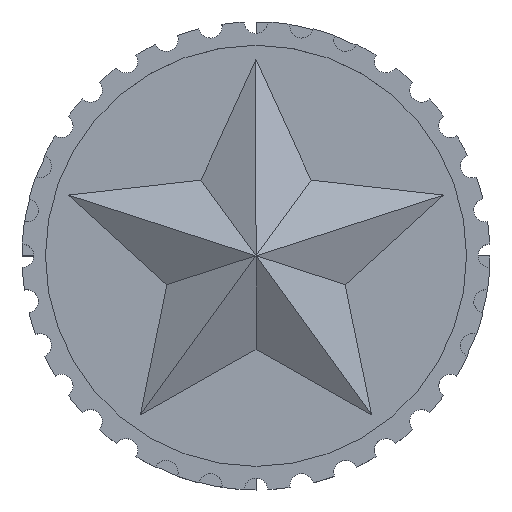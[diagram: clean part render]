
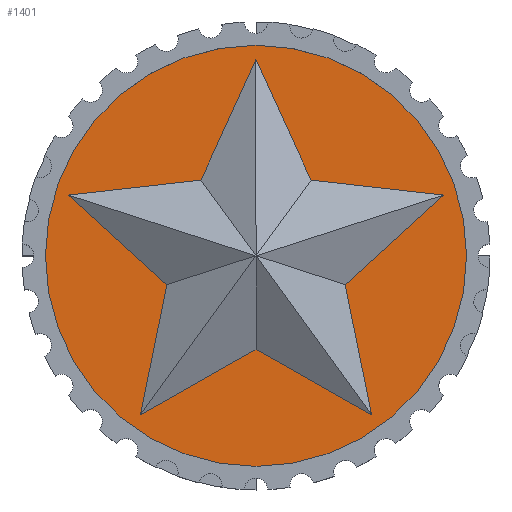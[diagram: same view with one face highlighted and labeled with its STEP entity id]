
A CAD part, top view. The second image highlights one B-rep face of the part: STEP entity #1401.
In plain terms, the highlighted planar face has unit normal (0, 0, 1).
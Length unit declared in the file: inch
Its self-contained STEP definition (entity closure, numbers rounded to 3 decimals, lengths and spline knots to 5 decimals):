
#27 = EDGE_CURVE ( 'NONE', #3067, #228, #1392, .T. ) ;
#35 = VERTEX_POINT ( 'NONE', #1314 ) ;
#119 = EDGE_CURVE ( 'NONE', #2326, #4335, #679, .T. ) ;
#147 = ORIENTED_EDGE ( 'NONE', *, *, #1856, .F. ) ;
#154 = EDGE_CURVE ( 'NONE', #560, #3881, #2661, .T. ) ;
#228 = VERTEX_POINT ( 'NONE', #1387 ) ;
#315 = LINE ( 'NONE', #2724, #3846 ) ;
#325 = CARTESIAN_POINT ( 'NONE',  ( 0., -0.25, 0.26063 ) ) ;
#347 = ORIENTED_EDGE ( 'NONE', *, *, #899, .F. ) ;
#560 = VERTEX_POINT ( 'NONE', #2029 ) ;
#591 = CARTESIAN_POINT ( 'NONE',  ( 0., 0.52533, 0.26063 ) ) ;
#642 = CIRCLE ( 'NONE', #1110, 0.5625 ) ;
#679 = LINE ( 'NONE', #2594, #3251 ) ;
#681 = DIRECTION ( 'NONE',  ( 0.738, -0.675, 0. ) ) ;
#683 = LINE ( 'NONE', #2772, #3199 ) ;
#722 = CARTESIAN_POINT ( 'NONE',  ( 0., 0., 0.26063 ) ) ;
#756 = EDGE_CURVE ( 'NONE', #1825, #560, #683, .T. ) ;
#802 = LINE ( 'NONE', #1806, #2503 ) ;
#899 = EDGE_CURVE ( 'NONE', #1241, #3067, #802, .T. ) ;
#919 = ORIENTED_EDGE ( 'NONE', *, *, #3669, .F. ) ;
#945 = CARTESIAN_POINT ( 'NONE',  ( -0.14695, 0.20225, 0.26063 ) ) ;
#970 = DIRECTION ( 'NONE',  ( -0.414, -0.91, 0. ) ) ;
#1079 = VERTEX_POINT ( 'NONE', #591 ) ;
#1110 = AXIS2_PLACEMENT_3D ( 'NONE', #722, #2523, #2877 ) ;
#1166 = CARTESIAN_POINT ( 'NONE',  ( 0., 0., 0.26063 ) ) ;
#1241 = VERTEX_POINT ( 'NONE', #325 ) ;
#1263 = LINE ( 'NONE', #2386, #4122 ) ;
#1279 = ORIENTED_EDGE ( 'NONE', *, *, #119, .F. ) ;
#1283 = VECTOR ( 'NONE', #3348, 39.37008 ) ;
#1301 = DIRECTION ( 'NONE',  ( -0.994, -0.112, 0. ) ) ;
#1314 = CARTESIAN_POINT ( 'NONE',  ( -0.14695, 0.20225, 0.26063 ) ) ;
#1351 = LINE ( 'NONE', #3572, #3530 ) ;
#1360 = LINE ( 'NONE', #945, #2111 ) ;
#1365 = CARTESIAN_POINT ( 'NONE',  ( 0.14695, 0.20225, 0.26063 ) ) ;
#1387 = CARTESIAN_POINT ( 'NONE',  ( 0.23776, -0.07725, 0.26063 ) ) ;
#1392 = LINE ( 'NONE', #2187, #1283 ) ;
#1401 = ADVANCED_FACE ( 'NONE', ( #3080, #1964 ), #3930, .T. ) ;
#1411 = ORIENTED_EDGE ( 'NONE', *, *, #756, .F. ) ;
#1482 = CIRCLE ( 'NONE', #3210, 0.5625 ) ;
#1547 = DIRECTION ( 'NONE',  ( -0.414, 0.91, 0. ) ) ;
#1581 = ORIENTED_EDGE ( 'NONE', *, *, #3782, .F. ) ;
#1721 = ORIENTED_EDGE ( 'NONE', *, *, #3905, .T. ) ;
#1752 = CARTESIAN_POINT ( 'NONE',  ( -0.30878, -0.425, 0.26063 ) ) ;
#1806 = CARTESIAN_POINT ( 'NONE',  ( 0., -0.25, 0.26063 ) ) ;
#1825 = VERTEX_POINT ( 'NONE', #2721 ) ;
#1856 = EDGE_CURVE ( 'NONE', #3881, #1241, #1263, .T. ) ;
#1857 = DIRECTION ( 'NONE',  ( 0., 0., 1. ) ) ;
#1885 = CARTESIAN_POINT ( 'NONE',  ( -0.5625, 0., 0.26063 ) ) ;
#1895 = EDGE_CURVE ( 'NONE', #2532, #3232, #1482, .T. ) ;
#1964 = FACE_BOUND ( 'NONE', #3190, .T. ) ;
#2029 = CARTESIAN_POINT ( 'NONE',  ( -0.23776, -0.07725, 0.26063 ) ) ;
#2111 = VECTOR ( 'NONE', #1301, 39.37008 ) ;
#2187 = CARTESIAN_POINT ( 'NONE',  ( 0.30878, -0.425, 0.26063 ) ) ;
#2238 = EDGE_CURVE ( 'NONE', #35, #1825, #1360, .T. ) ;
#2261 = EDGE_LOOP ( 'NONE', ( #1721, #3886 ) ) ;
#2326 = VERTEX_POINT ( 'NONE', #4056 ) ;
#2386 = CARTESIAN_POINT ( 'NONE',  ( -0.30878, -0.425, 0.26063 ) ) ;
#2442 = DIRECTION ( 'NONE',  ( 0.738, 0.675, 0. ) ) ;
#2501 = DIRECTION ( 'NONE',  ( 0., 0., 1. ) ) ;
#2503 = VECTOR ( 'NONE', #4166, 39.37008 ) ;
#2504 = DIRECTION ( 'NONE',  ( 1., 0., 0. ) ) ;
#2523 = DIRECTION ( 'NONE',  ( 0., 0., 1. ) ) ;
#2532 = VERTEX_POINT ( 'NONE', #1885 ) ;
#2594 = CARTESIAN_POINT ( 'NONE',  ( 0.49962, 0.16234, 0.26063 ) ) ;
#2661 = LINE ( 'NONE', #3595, #3941 ) ;
#2721 = CARTESIAN_POINT ( 'NONE',  ( -0.49962, 0.16234, 0.26063 ) ) ;
#2724 = CARTESIAN_POINT ( 'NONE',  ( 0.23776, -0.07725, 0.26063 ) ) ;
#2772 = CARTESIAN_POINT ( 'NONE',  ( -0.49962, 0.16234, 0.26063 ) ) ;
#2877 = DIRECTION ( 'NONE',  ( 1., 0., 0. ) ) ;
#3067 = VERTEX_POINT ( 'NONE', #3925 ) ;
#3080 = FACE_OUTER_BOUND ( 'NONE', #2261, .T. ) ;
#3190 = EDGE_LOOP ( 'NONE', ( #147, #4409, #1411, #3560, #1581, #919, #1279, #3927, #4251, #347 ) ) ;
#3191 = CARTESIAN_POINT ( 'NONE',  ( 0., 0., 0.26063 ) ) ;
#3199 = VECTOR ( 'NONE', #681, 39.37008 ) ;
#3210 = AXIS2_PLACEMENT_3D ( 'NONE', #3191, #2501, #3527 ) ;
#3232 = VERTEX_POINT ( 'NONE', #4276 ) ;
#3251 = VECTOR ( 'NONE', #3259, 39.37008 ) ;
#3259 = DIRECTION ( 'NONE',  ( -0.994, 0.112, 0. ) ) ;
#3315 = CARTESIAN_POINT ( 'NONE',  ( 0., 0.52533, 0.26063 ) ) ;
#3348 = DIRECTION ( 'NONE',  ( -0.2, 0.98, 0. ) ) ;
#3527 = DIRECTION ( 'NONE',  ( 1., 0., 0. ) ) ;
#3530 = VECTOR ( 'NONE', #1547, 39.37008 ) ;
#3560 = ORIENTED_EDGE ( 'NONE', *, *, #2238, .F. ) ;
#3572 = CARTESIAN_POINT ( 'NONE',  ( 0.14695, 0.20225, 0.26063 ) ) ;
#3584 = LINE ( 'NONE', #3315, #3850 ) ;
#3595 = CARTESIAN_POINT ( 'NONE',  ( -0.23776, -0.07725, 0.26063 ) ) ;
#3669 = EDGE_CURVE ( 'NONE', #4335, #1079, #1351, .T. ) ;
#3744 = DIRECTION ( 'NONE',  ( -0.2, -0.98, 0. ) ) ;
#3782 = EDGE_CURVE ( 'NONE', #1079, #35, #3584, .T. ) ;
#3846 = VECTOR ( 'NONE', #2442, 39.37008 ) ;
#3850 = VECTOR ( 'NONE', #970, 39.37008 ) ;
#3881 = VERTEX_POINT ( 'NONE', #1752 ) ;
#3886 = ORIENTED_EDGE ( 'NONE', *, *, #1895, .T. ) ;
#3905 = EDGE_CURVE ( 'NONE', #3232, #2532, #642, .T. ) ;
#3925 = CARTESIAN_POINT ( 'NONE',  ( 0.30878, -0.425, 0.26063 ) ) ;
#3927 = ORIENTED_EDGE ( 'NONE', *, *, #4403, .F. ) ;
#3930 = PLANE ( 'NONE',  #4315 ) ;
#3941 = VECTOR ( 'NONE', #3744, 39.37008 ) ;
#4056 = CARTESIAN_POINT ( 'NONE',  ( 0.49962, 0.16234, 0.26063 ) ) ;
#4102 = DIRECTION ( 'NONE',  ( 0.87, 0.493, 0. ) ) ;
#4122 = VECTOR ( 'NONE', #4102, 39.37008 ) ;
#4166 = DIRECTION ( 'NONE',  ( 0.87, -0.493, 0. ) ) ;
#4251 = ORIENTED_EDGE ( 'NONE', *, *, #27, .F. ) ;
#4276 = CARTESIAN_POINT ( 'NONE',  ( 0.5625, 0., 0.26063 ) ) ;
#4315 = AXIS2_PLACEMENT_3D ( 'NONE', #1166, #1857, #2504 ) ;
#4335 = VERTEX_POINT ( 'NONE', #1365 ) ;
#4403 = EDGE_CURVE ( 'NONE', #228, #2326, #315, .T. ) ;
#4409 = ORIENTED_EDGE ( 'NONE', *, *, #154, .F. ) ;
